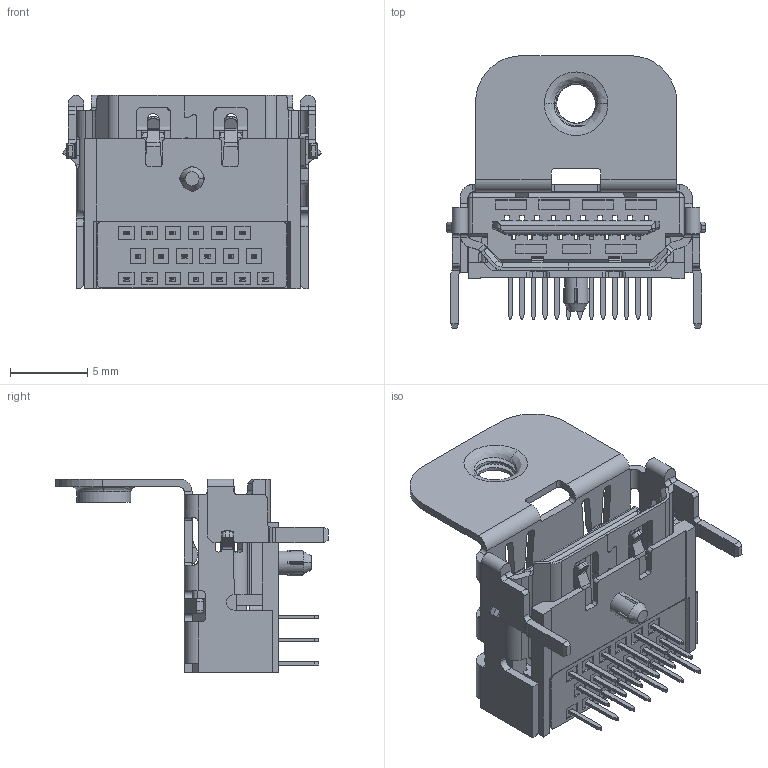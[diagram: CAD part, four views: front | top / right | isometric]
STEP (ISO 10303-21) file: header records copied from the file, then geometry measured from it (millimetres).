
FILE_DESCRIPTION (( 'STEP AP214' ), '1' );
FILE_NAME ('694B119-127-611.STEP', '2021-01-13T14:03:13', ( '' ), ( '' ), 'SwSTEP 2.0', 'SolidWorks 2020', '' );
FILE_SCHEMA (( 'AUTOMOTIVE_DESIGN' ));
Length unit declared in the file: millimetre
Products named in the file (23): Contact 7 694B119-X27-611; Insulator 694B119-X27-611; Contact 9 694B119-X27-611; Contact 1 694B119-X27-611; Contact 13 694B119-X27-611; Contact 19 694B119-X27-611; Contact 14 694B119-X27-611; Contact 4 694B119-X27-611; Contact 11 694B119-X27-611; Contact 2 694B119-X27-611; Contact 6 694B119-X27-611; Contact 16 694B119-X27-611; Contact 18 694B119-X27-611; Shell 694B119-X27-611; Contact 3 694B119-X27-611; Insulator2 694B119-X27-611; Contact 15 694B119-X27-611; Contact 8 694B119-X27-611; 694B119-127-611; Contact 17 694B119-X27-611; Contact 10 694B119-X27-611; Contact 12 694B119-X27-611; Contact 5 694B119-X27-611
Assembly tree (22 placements, depth 2):
  694B119-127-611
    Insulator 694B119-X27-611
    Contact 2 694B119-X27-611
    Contact 4 694B119-X27-611
    Contact 6 694B119-X27-611
    Contact 8 694B119-X27-611
    Contact 10 694B119-X27-611
    Contact 12 694B119-X27-611
    Contact 14 694B119-X27-611
    Contact 16 694B119-X27-611
    Contact 18 694B119-X27-611
    Contact 1 694B119-X27-611
    Contact 3 694B119-X27-611
    Contact 5 694B119-X27-611
    Contact 7 694B119-X27-611
    Contact 9 694B119-X27-611
    Contact 11 694B119-X27-611
    Contact 13 694B119-X27-611
    Contact 15 694B119-X27-611
    Contact 17 694B119-X27-611
    Contact 19 694B119-X27-611
    Insulator2 694B119-X27-611
    Shell 694B119-X27-611
Bounding box: 16.75 x 17.6 x 12.5 mm (x, y, z)
Volume: 596.6 mm3; surface area: 2570 mm2
Topology: 22 solids, 22 shells, 2042 faces, 5758 edges, 3728 vertices
Faces by surface type: plane 1664, cylinder 326, bspline 48, cone 4
Entity records: 68680 total; most frequent: CARTESIAN_POINT 15192, ORIENTED_EDGE 11514, DIRECTION 10022, EDGE_CURVE 5757, VECTOR 4928, LINE 4928, VERTEX_POINT 3729, AXIS2_PLACEMENT_3D 2547
